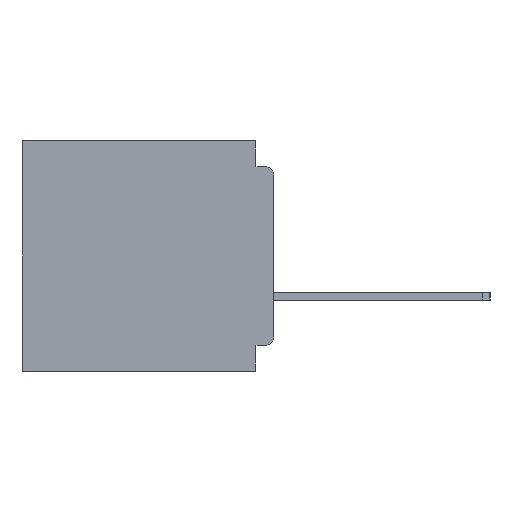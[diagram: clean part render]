
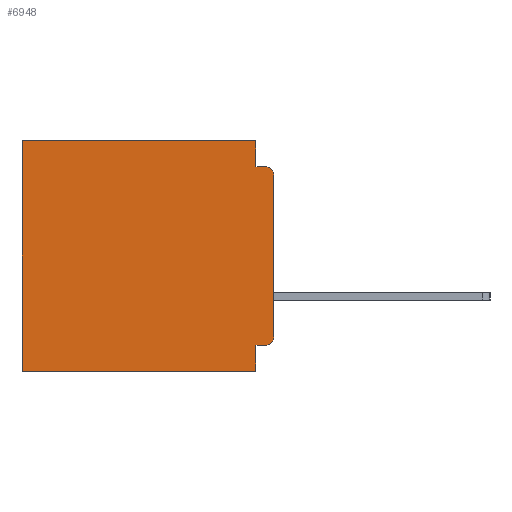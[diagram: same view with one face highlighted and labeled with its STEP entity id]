
A CAD part, left-side view. The second image highlights one B-rep face of the part: STEP entity #6948.
In plain terms, the highlighted planar face has unit normal (-1, 0, 0).
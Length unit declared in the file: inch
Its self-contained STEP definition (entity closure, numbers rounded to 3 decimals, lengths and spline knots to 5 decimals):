
#1841 = ORIENTED_EDGE ( 'NONE', *, *, #2775, .F. ) ;
#2775 = EDGE_CURVE ( 'NONE', #59870, #9327, #64230, .T. ) ;
#2887 = LINE ( 'NONE', #59882, #41884 ) ;
#2939 = CARTESIAN_POINT ( 'NONE',  ( 0.3, 0.437, -0.4 ) ) ;
#4706 = EDGE_CURVE ( 'NONE', #9327, #24065, #60669, .T. ) ;
#5068 = CARTESIAN_POINT ( 'NONE',  ( 0.3, 0.031, -0.355 ) ) ;
#6362 = EDGE_CURVE ( 'NONE', #52903, #16720, #34934, .T. ) ;
#6948 = ADVANCED_FACE ( 'NONE', ( #54002 ), #13949, .F. ) ;
#8613 = ORIENTED_EDGE ( 'NONE', *, *, #25568, .F. ) ;
#8671 = VERTEX_POINT ( 'NONE', #24375 ) ;
#8920 = LINE ( 'NONE', #10293, #61466 ) ;
#9212 = DIRECTION ( 'NONE',  ( 0., 0., -1. ) ) ;
#9327 = VERTEX_POINT ( 'NONE', #5068 ) ;
#9555 = CARTESIAN_POINT ( 'NONE',  ( 0.3, 0.015, -0.06 ) ) ;
#10293 = CARTESIAN_POINT ( 'NONE',  ( 0.3, 0.031, 0. ) ) ;
#10357 = EDGE_LOOP ( 'NONE', ( #43110, #34461, #53086, #15599, #40821, #39282, #8613, #10620, #1841, #55694 ) ) ;
#10620 = ORIENTED_EDGE ( 'NONE', *, *, #4706, .F. ) ;
#10697 = VECTOR ( 'NONE', #44228, 39.37008 ) ;
#13524 = EDGE_CURVE ( 'NONE', #19118, #59085, #8920, .T. ) ;
#13949 = PLANE ( 'NONE',  #27605 ) ;
#14692 = DIRECTION ( 'NONE',  ( 0., 0., -1. ) ) ;
#15599 = ORIENTED_EDGE ( 'NONE', *, *, #13524, .F. ) ;
#16720 = VERTEX_POINT ( 'NONE', #62575 ) ;
#17294 = VERTEX_POINT ( 'NONE', #56783 ) ;
#18386 = DIRECTION ( 'NONE',  ( 0., 0., -1. ) ) ;
#19118 = VERTEX_POINT ( 'NONE', #53821 ) ;
#21716 = VECTOR ( 'NONE', #9212, 39.37008 ) ;
#23720 = VECTOR ( 'NONE', #58353, 39.37008 ) ;
#24065 = VERTEX_POINT ( 'NONE', #44682 ) ;
#24227 = DIRECTION ( 'NONE',  ( 1., 0., 0. ) ) ;
#24375 = CARTESIAN_POINT ( 'NONE',  ( 0.3, 0.437, 0. ) ) ;
#25315 = AXIS2_PLACEMENT_3D ( 'NONE', #27489, #63038, #32560 ) ;
#25568 = EDGE_CURVE ( 'NONE', #24065, #17294, #51335, .T. ) ;
#27489 = CARTESIAN_POINT ( 'NONE',  ( 0.3, 0.015, -0.34 ) ) ;
#27605 = AXIS2_PLACEMENT_3D ( 'NONE', #49337, #24227, #59769 ) ;
#29411 = CARTESIAN_POINT ( 'NONE',  ( 0.3, 0.031, -0.045 ) ) ;
#30279 = CARTESIAN_POINT ( 'NONE',  ( 0.3, 0.031, -0.4 ) ) ;
#30559 = DIRECTION ( 'NONE',  ( 0., 0., -1. ) ) ;
#32248 = EDGE_CURVE ( 'NONE', #59870, #54875, #56831, .T. ) ;
#32560 = DIRECTION ( 'NONE',  ( 0., 0., -1. ) ) ;
#32597 = AXIS2_PLACEMENT_3D ( 'NONE', #9555, #45130, #14692 ) ;
#34461 = ORIENTED_EDGE ( 'NONE', *, *, #6362, .T. ) ;
#34683 = CARTESIAN_POINT ( 'NONE',  ( 0.3, 0., -0.34 ) ) ;
#34934 = CIRCLE ( 'NONE', #32597, 0.015 ) ;
#35350 = DIRECTION ( 'NONE',  ( 0., 0., -1. ) ) ;
#35409 = CARTESIAN_POINT ( 'NONE',  ( 0.3, 0., -0.355 ) ) ;
#36467 = VECTOR ( 'NONE', #56141, 39.37008 ) ;
#39103 = CARTESIAN_POINT ( 'NONE',  ( 0.3, 0., -0.4 ) ) ;
#39282 = ORIENTED_EDGE ( 'NONE', *, *, #58279, .T. ) ;
#40821 = ORIENTED_EDGE ( 'NONE', *, *, #65846, .T. ) ;
#41884 = VECTOR ( 'NONE', #64926, 39.37008 ) ;
#43110 = ORIENTED_EDGE ( 'NONE', *, *, #51017, .F. ) ;
#44228 = DIRECTION ( 'NONE',  ( 0., 1., 0. ) ) ;
#44682 = CARTESIAN_POINT ( 'NONE',  ( 0.3, 0.031, -0.4 ) ) ;
#44983 = VECTOR ( 'NONE', #18386, 39.37008 ) ;
#45130 = DIRECTION ( 'NONE',  ( -1., 0., 0. ) ) ;
#45506 = VECTOR ( 'NONE', #35350, 39.37008 ) ;
#47628 = EDGE_CURVE ( 'NONE', #59085, #16720, #2887, .T. ) ;
#48187 = LINE ( 'NONE', #2939, #44983 ) ;
#49337 = CARTESIAN_POINT ( 'NONE',  ( 0.3, 0., -0.4 ) ) ;
#49520 = CARTESIAN_POINT ( 'NONE',  ( 0.3, 0., -0.4 ) ) ;
#50338 = LINE ( 'NONE', #49520, #21716 ) ;
#51017 = EDGE_CURVE ( 'NONE', #52903, #54875, #50338, .T. ) ;
#51027 = CARTESIAN_POINT ( 'NONE',  ( 0.3, 0., 0. ) ) ;
#51335 = LINE ( 'NONE', #39103, #10697 ) ;
#52903 = VERTEX_POINT ( 'NONE', #59169 ) ;
#53086 = ORIENTED_EDGE ( 'NONE', *, *, #47628, .F. ) ;
#53242 = LINE ( 'NONE', #51027, #36467 ) ;
#53821 = CARTESIAN_POINT ( 'NONE',  ( 0.3, 0.031, 0. ) ) ;
#54002 = FACE_OUTER_BOUND ( 'NONE', #10357, .T. ) ;
#54875 = VERTEX_POINT ( 'NONE', #34683 ) ;
#55694 = ORIENTED_EDGE ( 'NONE', *, *, #32248, .T. ) ;
#56141 = DIRECTION ( 'NONE',  ( 0., 1., 0. ) ) ;
#56783 = CARTESIAN_POINT ( 'NONE',  ( 0.3, 0.437, -0.4 ) ) ;
#56831 = CIRCLE ( 'NONE', #25315, 0.015 ) ;
#56904 = CARTESIAN_POINT ( 'NONE',  ( 0.3, 0.015, -0.355 ) ) ;
#58279 = EDGE_CURVE ( 'NONE', #8671, #17294, #48187, .T. ) ;
#58353 = DIRECTION ( 'NONE',  ( 0., 1., 0. ) ) ;
#59085 = VERTEX_POINT ( 'NONE', #29411 ) ;
#59169 = CARTESIAN_POINT ( 'NONE',  ( 0.3, 0., -0.06 ) ) ;
#59769 = DIRECTION ( 'NONE',  ( 0., 0., -1. ) ) ;
#59870 = VERTEX_POINT ( 'NONE', #56904 ) ;
#59882 = CARTESIAN_POINT ( 'NONE',  ( 0.3, 0., -0.045 ) ) ;
#60669 = LINE ( 'NONE', #30279, #45506 ) ;
#61466 = VECTOR ( 'NONE', #30559, 39.37008 ) ;
#62575 = CARTESIAN_POINT ( 'NONE',  ( 0.3, 0.015, -0.045 ) ) ;
#63038 = DIRECTION ( 'NONE',  ( -1., 0., 0. ) ) ;
#64230 = LINE ( 'NONE', #35409, #23720 ) ;
#64926 = DIRECTION ( 'NONE',  ( 0., -1., 0. ) ) ;
#65846 = EDGE_CURVE ( 'NONE', #19118, #8671, #53242, .T. ) ;
